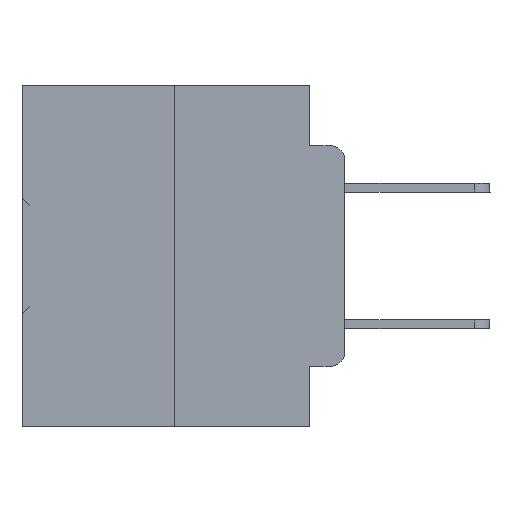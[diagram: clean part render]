
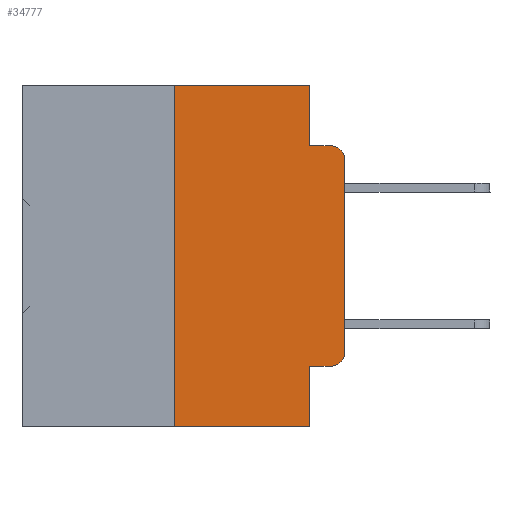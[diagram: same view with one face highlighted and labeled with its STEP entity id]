
A CAD part, left-side view. The second image highlights one B-rep face of the part: STEP entity #34777.
In plain terms, the highlighted planar face has unit normal (-1, 0, 0).
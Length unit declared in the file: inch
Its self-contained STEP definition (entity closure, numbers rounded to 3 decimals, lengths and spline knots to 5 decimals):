
#57 = AXIS2_PLACEMENT_3D ( 'NONE', #7262, #28444, #10378 ) ;
#139 = CARTESIAN_POINT ( 'NONE',  ( 0., 0.051, -0.4115 ) ) ;
#290 = DIRECTION ( 'NONE',  ( 0., 0., -1. ) ) ;
#704 = EDGE_CURVE ( 'NONE', #37879, #21885, #23925, .T. ) ;
#716 = ORIENTED_EDGE ( 'NONE', *, *, #704, .T. ) ;
#1194 = ORIENTED_EDGE ( 'NONE', *, *, #11389, .T. ) ;
#3091 = EDGE_CURVE ( 'NONE', #30014, #13912, #24582, .T. ) ;
#3221 = DIRECTION ( 'NONE',  ( 0., 0., -1. ) ) ;
#4692 = CARTESIAN_POINT ( 'NONE',  ( 0., 0., 0. ) ) ;
#5248 = CARTESIAN_POINT ( 'NONE',  ( 0., 0.051, -0.0885 ) ) ;
#7261 = EDGE_CURVE ( 'NONE', #13912, #10792, #8142, .T. ) ;
#7262 = CARTESIAN_POINT ( 'NONE',  ( 0., 0.02, -0.1085 ) ) ;
#7735 = CARTESIAN_POINT ( 'NONE',  ( 0., 0.051, 0. ) ) ;
#7794 = VECTOR ( 'NONE', #14479, 39.37008 ) ;
#7895 = VERTEX_POINT ( 'NONE', #14809 ) ;
#8142 = LINE ( 'NONE', #5248, #39146 ) ;
#8489 = VECTOR ( 'NONE', #3221, 39.37008 ) ;
#8875 = CIRCLE ( 'NONE', #57, 0.02 ) ;
#9268 = CARTESIAN_POINT ( 'NONE',  ( 0., 0.25, -0.5 ) ) ;
#9806 = PLANE ( 'NONE',  #20557 ) ;
#10020 = ORIENTED_EDGE ( 'NONE', *, *, #32291, .T. ) ;
#10171 = EDGE_CURVE ( 'NONE', #15814, #30014, #35308, .T. ) ;
#10378 = DIRECTION ( 'NONE',  ( 0., 0., -1. ) ) ;
#10609 = CARTESIAN_POINT ( 'NONE',  ( 0., 0.473, -0.5 ) ) ;
#10792 = VERTEX_POINT ( 'NONE', #13583 ) ;
#10855 = CARTESIAN_POINT ( 'NONE',  ( 0., 0.02, -0.4115 ) ) ;
#11389 = EDGE_CURVE ( 'NONE', #38214, #10792, #8875, .T. ) ;
#11427 = ORIENTED_EDGE ( 'NONE', *, *, #7261, .F. ) ;
#11836 = EDGE_LOOP ( 'NONE', ( #24658, #1194, #11427, #35384, #37229, #14244, #716, #25130, #10020, #11917 ) ) ;
#11917 = ORIENTED_EDGE ( 'NONE', *, *, #30287, .T. ) ;
#12420 = CARTESIAN_POINT ( 'NONE',  ( 0., 0.051, -0.4115 ) ) ;
#13195 = LINE ( 'NONE', #37313, #27358 ) ;
#13583 = CARTESIAN_POINT ( 'NONE',  ( 0., 0.02, -0.0885 ) ) ;
#13776 = DIRECTION ( 'NONE',  ( 0., 0., 1. ) ) ;
#13832 = LINE ( 'NONE', #4692, #30777 ) ;
#13912 = VERTEX_POINT ( 'NONE', #24633 ) ;
#14244 = ORIENTED_EDGE ( 'NONE', *, *, #38267, .F. ) ;
#14479 = DIRECTION ( 'NONE',  ( 0., -1., 0. ) ) ;
#14809 = CARTESIAN_POINT ( 'NONE',  ( 0., 0., -0.3915 ) ) ;
#15428 = EDGE_CURVE ( 'NONE', #7895, #38214, #13832, .T. ) ;
#15814 = VERTEX_POINT ( 'NONE', #36580 ) ;
#16276 = VECTOR ( 'NONE', #18617, 39.37008 ) ;
#16402 = VERTEX_POINT ( 'NONE', #12420 ) ;
#16677 = DIRECTION ( 'NONE',  ( 0., -1., 0. ) ) ;
#17883 = VERTEX_POINT ( 'NONE', #10855 ) ;
#18617 = DIRECTION ( 'NONE',  ( 0., -1., 0. ) ) ;
#18753 = DIRECTION ( 'NONE',  ( -1., 0., 0. ) ) ;
#19409 = VECTOR ( 'NONE', #16677, 39.37008 ) ;
#19429 = DIRECTION ( 'NONE',  ( 0., 0., -1. ) ) ;
#20557 = AXIS2_PLACEMENT_3D ( 'NONE', #24868, #21867, #30856 ) ;
#21867 = DIRECTION ( 'NONE',  ( 1., 0., 0. ) ) ;
#21885 = VERTEX_POINT ( 'NONE', #35690 ) ;
#23001 = CARTESIAN_POINT ( 'NONE',  ( 0., 0., -0.1085 ) ) ;
#23925 = LINE ( 'NONE', #10609, #7794 ) ;
#24012 = CARTESIAN_POINT ( 'NONE',  ( 0., 0.051, 0. ) ) ;
#24582 = LINE ( 'NONE', #24012, #8489 ) ;
#24633 = CARTESIAN_POINT ( 'NONE',  ( 0., 0.051, -0.0885 ) ) ;
#24658 = ORIENTED_EDGE ( 'NONE', *, *, #15428, .T. ) ;
#24868 = CARTESIAN_POINT ( 'NONE',  ( 0., 0.473, 0. ) ) ;
#25130 = ORIENTED_EDGE ( 'NONE', *, *, #36270, .F. ) ;
#26279 = DIRECTION ( 'NONE',  ( 0., 0., 1. ) ) ;
#27358 = VECTOR ( 'NONE', #19429, 39.37008 ) ;
#27660 = VECTOR ( 'NONE', #26279, 39.37008 ) ;
#28444 = DIRECTION ( 'NONE',  ( -1., 0., 0. ) ) ;
#30014 = VERTEX_POINT ( 'NONE', #7735 ) ;
#30287 = EDGE_CURVE ( 'NONE', #17883, #7895, #30804, .T. ) ;
#30777 = VECTOR ( 'NONE', #13776, 39.37008 ) ;
#30804 = CIRCLE ( 'NONE', #35704, 0.02 ) ;
#30856 = DIRECTION ( 'NONE',  ( 0., 0., -1. ) ) ;
#32291 = EDGE_CURVE ( 'NONE', #16402, #17883, #33186, .T. ) ;
#33186 = LINE ( 'NONE', #139, #16276 ) ;
#33980 = FACE_OUTER_BOUND ( 'NONE', #11836, .T. ) ;
#34777 = ADVANCED_FACE ( 'NONE', ( #33980 ), #9806, .F. ) ;
#35308 = LINE ( 'NONE', #37605, #19409 ) ;
#35384 = ORIENTED_EDGE ( 'NONE', *, *, #3091, .F. ) ;
#35453 = DIRECTION ( 'NONE',  ( 0., -1., 0. ) ) ;
#35555 = LINE ( 'NONE', #38101, #27660 ) ;
#35690 = CARTESIAN_POINT ( 'NONE',  ( 0., 0.051, -0.5 ) ) ;
#35704 = AXIS2_PLACEMENT_3D ( 'NONE', #36661, #18753, #290 ) ;
#36270 = EDGE_CURVE ( 'NONE', #16402, #21885, #13195, .T. ) ;
#36580 = CARTESIAN_POINT ( 'NONE',  ( 0., 0.25, 0. ) ) ;
#36661 = CARTESIAN_POINT ( 'NONE',  ( 0., 0.02, -0.3915 ) ) ;
#37229 = ORIENTED_EDGE ( 'NONE', *, *, #10171, .F. ) ;
#37313 = CARTESIAN_POINT ( 'NONE',  ( 0., 0.051, 0. ) ) ;
#37605 = CARTESIAN_POINT ( 'NONE',  ( 0., 0.473, 0. ) ) ;
#37879 = VERTEX_POINT ( 'NONE', #9268 ) ;
#38101 = CARTESIAN_POINT ( 'NONE',  ( 0., 0.25, 0. ) ) ;
#38214 = VERTEX_POINT ( 'NONE', #23001 ) ;
#38267 = EDGE_CURVE ( 'NONE', #37879, #15814, #35555, .T. ) ;
#39146 = VECTOR ( 'NONE', #35453, 39.37008 ) ;
